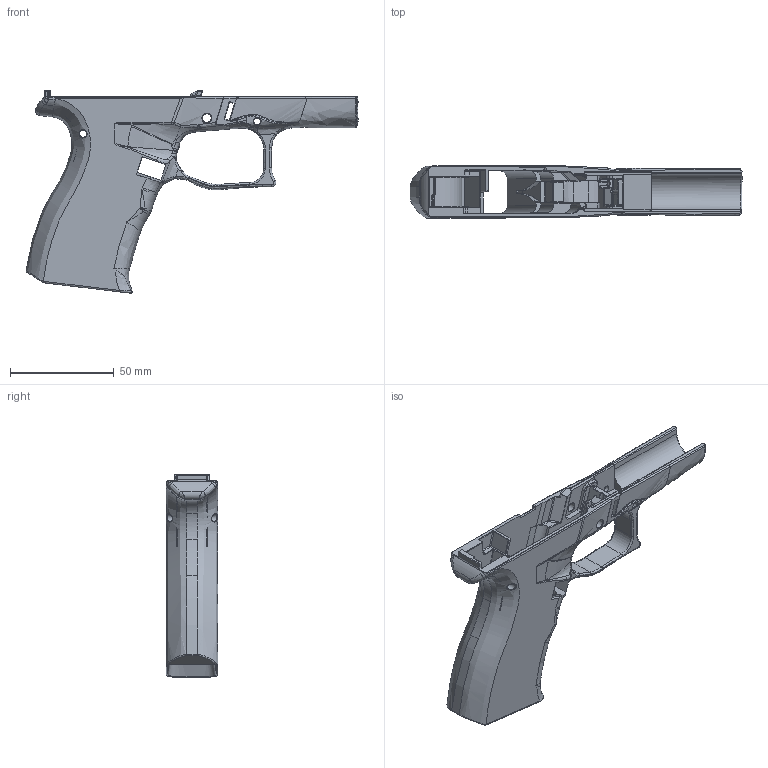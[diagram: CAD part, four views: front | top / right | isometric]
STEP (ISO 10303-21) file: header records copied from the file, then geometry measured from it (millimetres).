
FILE_DESCRIPTION(/* description */ ('Unknown'),/* implementation_level */ '2;1');
FILE_NAME(/* name */ 'Frame 43X',/* time_stamp */ '2022-06-13T16:30:27-05:00',/* author */ ('Unknown'),/* organization */ ('Unknown'),/* preprocessor_version */ 'ST-DEVELOPER v18.1',/* originating_system */ 'Solid Edge',/* authorisation */ 'Unknown');
FILE_SCHEMA (('AUTOMOTIVE_DESIGN {1 0 10303 214 3 1 1}'));
Length unit declared in the file: millimetre
Products named in the file (1): Frame 43X
Bounding box: 160.07 x 25 x 97.66 mm (x, y, z)
Volume: 51749 mm3; surface area: 36190.7 mm2
Topology: 1 solids, 2 shells, 949 faces, 2507 edges, 1499 vertices
Faces by surface type: bspline 404, cylinder 258, plane 165, torus 77, sphere 30, cone 15
Full cylindrical faces by diameter (mm): 3.3 x2, 3.5 x3, 4.25 x2
Entity records: 47681 total; most frequent: CARTESIAN_POINT 28055, ORIENTED_EDGE 4860, DIRECTION 2946, EDGE_CURVE 2430, VERTEX_POINT 1490, B_SPLINE_CURVE_WITH_KNOTS 1173, AXIS2_PLACEMENT_3D 1146, EDGE_LOOP 978
